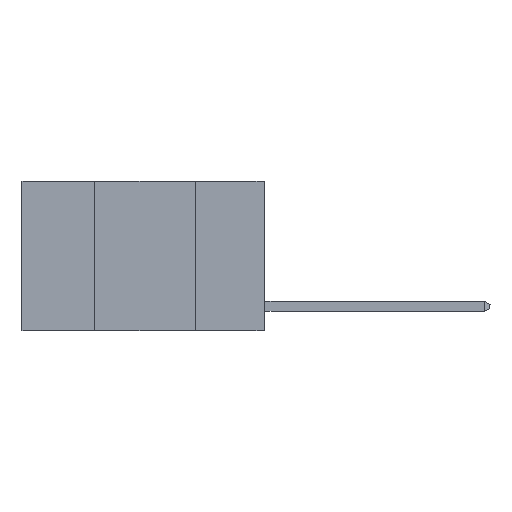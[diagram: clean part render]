
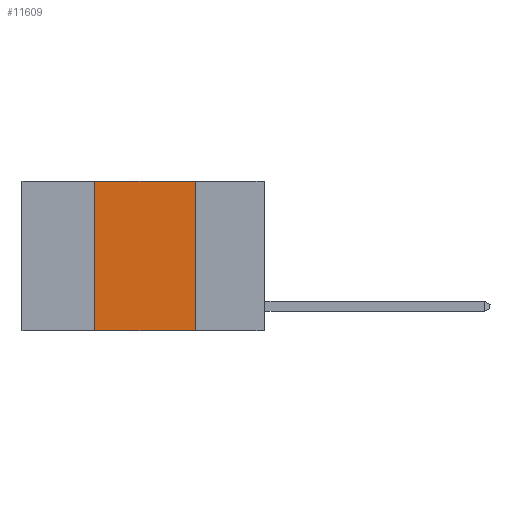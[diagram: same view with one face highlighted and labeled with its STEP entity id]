
A CAD part, left-side view. The second image highlights one B-rep face of the part: STEP entity #11609.
In plain terms, the highlighted planar face has unit normal (-1, 0, 0).
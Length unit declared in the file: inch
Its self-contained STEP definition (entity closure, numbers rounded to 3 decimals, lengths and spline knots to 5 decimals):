
#274 = VERTEX_POINT ( 'NONE', #9636 ) ;
#530 = DIRECTION ( 'NONE',  ( 0., 0., -1. ) ) ;
#1282 = VERTEX_POINT ( 'NONE', #7382 ) ;
#1288 = DIRECTION ( 'NONE',  ( 1., 0., 0. ) ) ;
#1590 = EDGE_LOOP ( 'NONE', ( #11465, #3703, #11152, #11534 ) ) ;
#2764 = VECTOR ( 'NONE', #530, 39.37008 ) ;
#2808 = CARTESIAN_POINT ( 'NONE',  ( 0., 0.17, 0. ) ) ;
#2963 = VERTEX_POINT ( 'NONE', #2808 ) ;
#3386 = PLANE ( 'NONE',  #4250 ) ;
#3629 = EDGE_CURVE ( 'NONE', #6970, #274, #4502, .T. ) ;
#3703 = ORIENTED_EDGE ( 'NONE', *, *, #9412, .F. ) ;
#3857 = FACE_OUTER_BOUND ( 'NONE', #1590, .T. ) ;
#3966 = CARTESIAN_POINT ( 'NONE',  ( 0., 0.6, 0. ) ) ;
#4250 = AXIS2_PLACEMENT_3D ( 'NONE', #9702, #1288, #10821 ) ;
#4502 = LINE ( 'NONE', #7157, #5675 ) ;
#5487 = LINE ( 'NONE', #6449, #6138 ) ;
#5675 = VECTOR ( 'NONE', #9402, 39.37008 ) ;
#5793 = EDGE_CURVE ( 'NONE', #2963, #274, #9748, .T. ) ;
#6138 = VECTOR ( 'NONE', #10497, 39.37008 ) ;
#6395 = LINE ( 'NONE', #3966, #8892 ) ;
#6449 = CARTESIAN_POINT ( 'NONE',  ( 0., 0.42, 0. ) ) ;
#6730 = EDGE_CURVE ( 'NONE', #6970, #1282, #5487, .T. ) ;
#6960 = CARTESIAN_POINT ( 'NONE',  ( 0., 0.17, 0. ) ) ;
#6970 = VERTEX_POINT ( 'NONE', #10680 ) ;
#7137 = DIRECTION ( 'NONE',  ( 0., -1., 0. ) ) ;
#7157 = CARTESIAN_POINT ( 'NONE',  ( 0., 0.6, -0.37 ) ) ;
#7382 = CARTESIAN_POINT ( 'NONE',  ( 0., 0.42, 0. ) ) ;
#8892 = VECTOR ( 'NONE', #7137, 39.37008 ) ;
#9402 = DIRECTION ( 'NONE',  ( 0., -1., 0. ) ) ;
#9412 = EDGE_CURVE ( 'NONE', #1282, #2963, #6395, .T. ) ;
#9636 = CARTESIAN_POINT ( 'NONE',  ( 0., 0.17, -0.37 ) ) ;
#9702 = CARTESIAN_POINT ( 'NONE',  ( 0., 0.6, 0. ) ) ;
#9748 = LINE ( 'NONE', #6960, #2764 ) ;
#10497 = DIRECTION ( 'NONE',  ( 0., 0., 1. ) ) ;
#10680 = CARTESIAN_POINT ( 'NONE',  ( 0., 0.42, -0.37 ) ) ;
#10821 = DIRECTION ( 'NONE',  ( 0., 0., -1. ) ) ;
#11152 = ORIENTED_EDGE ( 'NONE', *, *, #6730, .F. ) ;
#11465 = ORIENTED_EDGE ( 'NONE', *, *, #5793, .F. ) ;
#11534 = ORIENTED_EDGE ( 'NONE', *, *, #3629, .T. ) ;
#11609 = ADVANCED_FACE ( 'NONE', ( #3857 ), #3386, .F. ) ;
